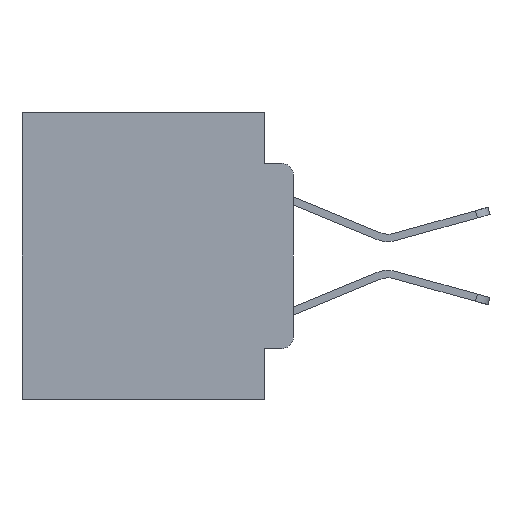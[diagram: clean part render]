
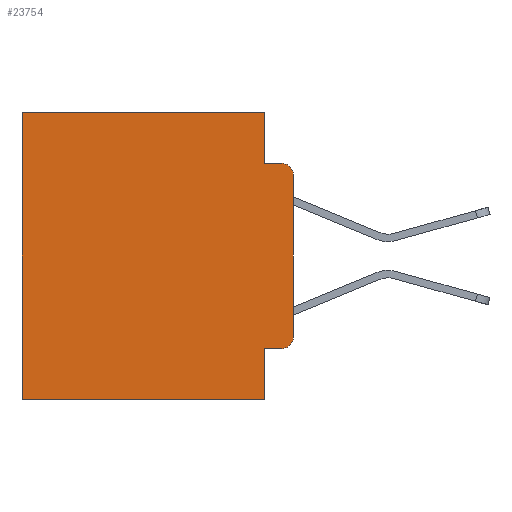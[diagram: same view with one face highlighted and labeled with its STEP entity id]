
A CAD part, left-side view. The second image highlights one B-rep face of the part: STEP entity #23754.
In plain terms, the highlighted planar face has unit normal (-1, 0, 0).
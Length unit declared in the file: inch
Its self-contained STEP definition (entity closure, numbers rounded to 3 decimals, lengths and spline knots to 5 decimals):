
#175 = VECTOR ( 'NONE', #1480, 39.37008 ) ;
#673 = VERTEX_POINT ( 'NONE', #9074 ) ;
#805 = ORIENTED_EDGE ( 'NONE', *, *, #3106, .F. ) ;
#940 = CARTESIAN_POINT ( 'NONE',  ( 0.298, 0., -0.1085 ) ) ;
#1480 = DIRECTION ( 'NONE',  ( 0., 0., -1. ) ) ;
#1674 = LINE ( 'NONE', #5301, #22505 ) ;
#1730 = EDGE_CURVE ( 'NONE', #21557, #19029, #22890, .T. ) ;
#2198 = CARTESIAN_POINT ( 'NONE',  ( 0.298, 0.473, 0. ) ) ;
#2383 = VERTEX_POINT ( 'NONE', #13593 ) ;
#3106 = EDGE_CURVE ( 'NONE', #22807, #2383, #10957, .T. ) ;
#3285 = VECTOR ( 'NONE', #24359, 39.37008 ) ;
#3600 = VERTEX_POINT ( 'NONE', #940 ) ;
#4337 = LINE ( 'NONE', #11661, #175 ) ;
#4791 = DIRECTION ( 'NONE',  ( 0., 0., -1. ) ) ;
#4947 = LINE ( 'NONE', #5389, #9107 ) ;
#5210 = CARTESIAN_POINT ( 'NONE',  ( 0.298, 0., 0. ) ) ;
#5271 = CARTESIAN_POINT ( 'NONE',  ( 0.298, 0.02, -0.1085 ) ) ;
#5301 = CARTESIAN_POINT ( 'NONE',  ( 0.298, 0., -0.5 ) ) ;
#5318 = CARTESIAN_POINT ( 'NONE',  ( 0.298, 0.051, -0.0885 ) ) ;
#5389 = CARTESIAN_POINT ( 'NONE',  ( 0.298, 0.051, -0.0885 ) ) ;
#5514 = VECTOR ( 'NONE', #17957, 39.37008 ) ;
#5757 = EDGE_CURVE ( 'NONE', #22807, #7918, #25711, .T. ) ;
#6545 = ORIENTED_EDGE ( 'NONE', *, *, #5757, .T. ) ;
#7331 = DIRECTION ( 'NONE',  ( 0., 0., -1. ) ) ;
#7467 = ORIENTED_EDGE ( 'NONE', *, *, #17949, .T. ) ;
#7918 = VERTEX_POINT ( 'NONE', #14058 ) ;
#8511 = CARTESIAN_POINT ( 'NONE',  ( 0.298, 0.02, -0.3915 ) ) ;
#8694 = CARTESIAN_POINT ( 'NONE',  ( 0.298, 0.051, 0. ) ) ;
#8717 = LINE ( 'NONE', #2198, #3285 ) ;
#8762 = ORIENTED_EDGE ( 'NONE', *, *, #25474, .F. ) ;
#8927 = CIRCLE ( 'NONE', #15396, 0.02 ) ;
#9074 = CARTESIAN_POINT ( 'NONE',  ( 0.298, 0.02, -0.0885 ) ) ;
#9107 = VECTOR ( 'NONE', #17552, 39.37008 ) ;
#9343 = DIRECTION ( 'NONE',  ( 1., 0., 0. ) ) ;
#9829 = EDGE_LOOP ( 'NONE', ( #18597, #18625, #10689, #12341, #22599, #11681, #8762, #805, #6545, #7467 ) ) ;
#9955 = EDGE_CURVE ( 'NONE', #3600, #673, #20639, .T. ) ;
#10577 = DIRECTION ( 'NONE',  ( 0., 0., -1. ) ) ;
#10689 = ORIENTED_EDGE ( 'NONE', *, *, #23821, .F. ) ;
#10957 = LINE ( 'NONE', #8694, #5514 ) ;
#11215 = PLANE ( 'NONE',  #13492 ) ;
#11437 = CARTESIAN_POINT ( 'NONE',  ( 0.298, 0.051, -0.4115 ) ) ;
#11661 = CARTESIAN_POINT ( 'NONE',  ( 0.298, 0., 0. ) ) ;
#11662 = VERTEX_POINT ( 'NONE', #23366 ) ;
#11681 = ORIENTED_EDGE ( 'NONE', *, *, #25141, .T. ) ;
#12230 = VERTEX_POINT ( 'NONE', #17504 ) ;
#12341 = ORIENTED_EDGE ( 'NONE', *, *, #1730, .F. ) ;
#12721 = EDGE_CURVE ( 'NONE', #3600, #12230, #4337, .T. ) ;
#12796 = CARTESIAN_POINT ( 'NONE',  ( 0.298, 0.051, -0.4115 ) ) ;
#13492 = AXIS2_PLACEMENT_3D ( 'NONE', #5210, #9343, #23307 ) ;
#13593 = CARTESIAN_POINT ( 'NONE',  ( 0.298, 0.051, -0.5 ) ) ;
#13632 = VECTOR ( 'NONE', #18160, 39.37008 ) ;
#14058 = CARTESIAN_POINT ( 'NONE',  ( 0.298, 0.02, -0.4115 ) ) ;
#14276 = LINE ( 'NONE', #16069, #13632 ) ;
#14625 = VERTEX_POINT ( 'NONE', #15721 ) ;
#14840 = DIRECTION ( 'NONE',  ( 0., -1., 0. ) ) ;
#15396 = AXIS2_PLACEMENT_3D ( 'NONE', #8511, #22544, #10577 ) ;
#15721 = CARTESIAN_POINT ( 'NONE',  ( 0.298, 0.473, 0. ) ) ;
#15783 = FACE_OUTER_BOUND ( 'NONE', #9829, .T. ) ;
#16069 = CARTESIAN_POINT ( 'NONE',  ( 0.298, 0., 0. ) ) ;
#17307 = CARTESIAN_POINT ( 'NONE',  ( 0.298, 0.051, 0. ) ) ;
#17472 = DIRECTION ( 'NONE',  ( 0., 1., 0. ) ) ;
#17504 = CARTESIAN_POINT ( 'NONE',  ( 0.298, 0., -0.3915 ) ) ;
#17552 = DIRECTION ( 'NONE',  ( 0., -1., 0. ) ) ;
#17949 = EDGE_CURVE ( 'NONE', #7918, #12230, #8927, .T. ) ;
#17957 = DIRECTION ( 'NONE',  ( 0., 0., -1. ) ) ;
#18160 = DIRECTION ( 'NONE',  ( 0., 1., 0. ) ) ;
#18597 = ORIENTED_EDGE ( 'NONE', *, *, #12721, .F. ) ;
#18625 = ORIENTED_EDGE ( 'NONE', *, *, #9955, .T. ) ;
#19029 = VERTEX_POINT ( 'NONE', #5318 ) ;
#19445 = DIRECTION ( 'NONE',  ( -1., 0., 0. ) ) ;
#19617 = AXIS2_PLACEMENT_3D ( 'NONE', #5271, #19445, #7331 ) ;
#20534 = VECTOR ( 'NONE', #14840, 39.37008 ) ;
#20639 = CIRCLE ( 'NONE', #19617, 0.02 ) ;
#21557 = VERTEX_POINT ( 'NONE', #24965 ) ;
#21707 = VECTOR ( 'NONE', #4791, 39.37008 ) ;
#21911 = EDGE_CURVE ( 'NONE', #21557, #14625, #14276, .T. ) ;
#22505 = VECTOR ( 'NONE', #17472, 39.37008 ) ;
#22544 = DIRECTION ( 'NONE',  ( -1., 0., 0. ) ) ;
#22599 = ORIENTED_EDGE ( 'NONE', *, *, #21911, .T. ) ;
#22807 = VERTEX_POINT ( 'NONE', #12796 ) ;
#22890 = LINE ( 'NONE', #17307, #21707 ) ;
#23307 = DIRECTION ( 'NONE',  ( 0., 0., -1. ) ) ;
#23366 = CARTESIAN_POINT ( 'NONE',  ( 0.298, 0.473, -0.5 ) ) ;
#23754 = ADVANCED_FACE ( 'NONE', ( #15783 ), #11215, .F. ) ;
#23821 = EDGE_CURVE ( 'NONE', #19029, #673, #4947, .T. ) ;
#24359 = DIRECTION ( 'NONE',  ( 0., 0., -1. ) ) ;
#24965 = CARTESIAN_POINT ( 'NONE',  ( 0.298, 0.051, 0. ) ) ;
#25141 = EDGE_CURVE ( 'NONE', #14625, #11662, #8717, .T. ) ;
#25474 = EDGE_CURVE ( 'NONE', #2383, #11662, #1674, .T. ) ;
#25711 = LINE ( 'NONE', #11437, #20534 ) ;
